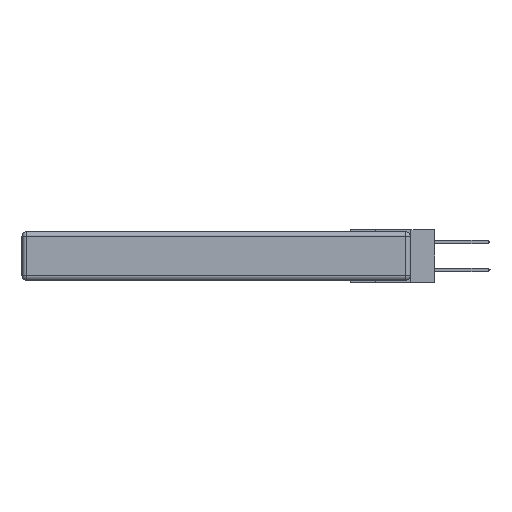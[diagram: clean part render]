
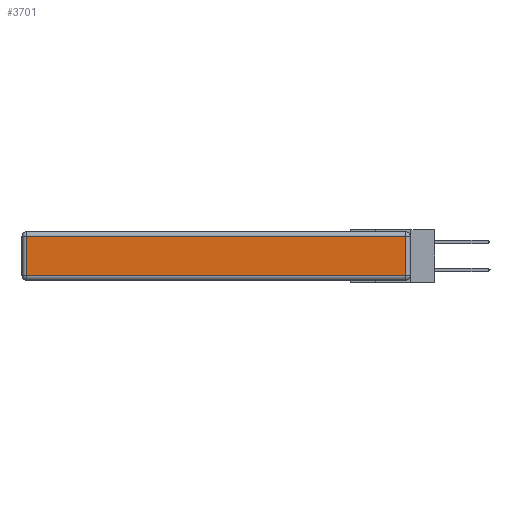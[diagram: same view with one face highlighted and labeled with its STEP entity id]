
A CAD part, left-side view. The second image highlights one B-rep face of the part: STEP entity #3701.
In plain terms, the highlighted planar face has unit normal (-1, 0, 0).
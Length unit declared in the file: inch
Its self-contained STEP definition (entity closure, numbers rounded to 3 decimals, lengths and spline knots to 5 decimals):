
#352 = VERTEX_POINT ( 'NONE', #20513 ) ;
#435 = EDGE_CURVE ( 'NONE', #352, #7866, #16406, .T. ) ;
#908 = LINE ( 'NONE', #11548, #8534 ) ;
#1029 = EDGE_CURVE ( 'NONE', #23471, #352, #12184, .T. ) ;
#1460 = CARTESIAN_POINT ( 'NONE',  ( 0., 0., -0.343 ) ) ;
#2121 = CARTESIAN_POINT ( 'NONE',  ( 0., 2.75, -0.03 ) ) ;
#3701 = ADVANCED_FACE ( 'NONE', ( #7270 ), #14726, .T. ) ;
#5064 = VECTOR ( 'NONE', #17762, 39.37008 ) ;
#5213 = ORIENTED_EDGE ( 'NONE', *, *, #435, .T. ) ;
#7270 = FACE_OUTER_BOUND ( 'NONE', #19614, .T. ) ;
#7866 = VERTEX_POINT ( 'NONE', #26858 ) ;
#8534 = VECTOR ( 'NONE', #9309, 39.37008 ) ;
#9260 = VECTOR ( 'NONE', #21425, 39.37008 ) ;
#9309 = DIRECTION ( 'NONE',  ( 0., -1., 0. ) ) ;
#11548 = CARTESIAN_POINT ( 'NONE',  ( 0., 0., -0.313 ) ) ;
#12184 = LINE ( 'NONE', #2121, #5064 ) ;
#14030 = ORIENTED_EDGE ( 'NONE', *, *, #1029, .T. ) ;
#14614 = DIRECTION ( 'NONE',  ( 0., 0., 1. ) ) ;
#14726 = PLANE ( 'NONE',  #26358 ) ;
#15433 = CARTESIAN_POINT ( 'NONE',  ( 0., 2.72, -0.343 ) ) ;
#16406 = LINE ( 'NONE', #15433, #31583 ) ;
#17762 = DIRECTION ( 'NONE',  ( 0., 1., 0. ) ) ;
#18488 = VERTEX_POINT ( 'NONE', #23080 ) ;
#19614 = EDGE_LOOP ( 'NONE', ( #23800, #30164, #14030, #5213 ) ) ;
#20513 = CARTESIAN_POINT ( 'NONE',  ( 0., 2.72, -0.03 ) ) ;
#21214 = CARTESIAN_POINT ( 'NONE',  ( 0., 0.03, -0.03 ) ) ;
#21425 = DIRECTION ( 'NONE',  ( 0., 0., 1. ) ) ;
#21460 = LINE ( 'NONE', #23805, #9260 ) ;
#23080 = CARTESIAN_POINT ( 'NONE',  ( 0., 0.03, -0.313 ) ) ;
#23104 = DIRECTION ( 'NONE',  ( 0., 0., -1. ) ) ;
#23471 = VERTEX_POINT ( 'NONE', #21214 ) ;
#23800 = ORIENTED_EDGE ( 'NONE', *, *, #24135, .T. ) ;
#23805 = CARTESIAN_POINT ( 'NONE',  ( 0., 0.03, -0.343 ) ) ;
#24135 = EDGE_CURVE ( 'NONE', #7866, #18488, #908, .T. ) ;
#26358 = AXIS2_PLACEMENT_3D ( 'NONE', #1460, #28393, #14614 ) ;
#26858 = CARTESIAN_POINT ( 'NONE',  ( 0., 2.72, -0.313 ) ) ;
#28393 = DIRECTION ( 'NONE',  ( -1., 0., 0. ) ) ;
#30164 = ORIENTED_EDGE ( 'NONE', *, *, #30346, .T. ) ;
#30346 = EDGE_CURVE ( 'NONE', #18488, #23471, #21460, .T. ) ;
#31583 = VECTOR ( 'NONE', #23104, 39.37008 ) ;
